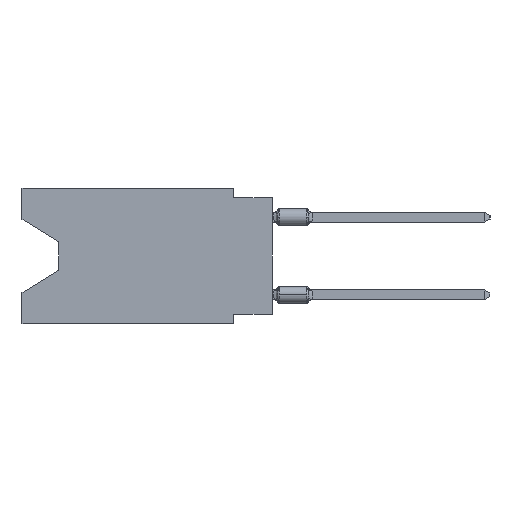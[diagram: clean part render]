
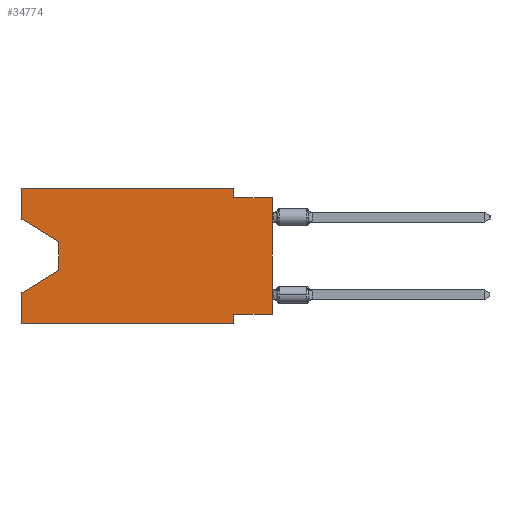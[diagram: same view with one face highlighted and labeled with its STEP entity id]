
A CAD part, left-side view. The second image highlights one B-rep face of the part: STEP entity #34774.
In plain terms, the highlighted planar face has unit normal (-1, 0, 0).
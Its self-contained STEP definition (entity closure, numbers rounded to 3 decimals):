
#83 = VERTEX_POINT ( 'NONE', #18799 ) ;
#604 = VECTOR ( 'NONE', #14084, 1000. ) ;
#1119 = CARTESIAN_POINT ( 'NONE',  ( 0., 0., -0.635 ) ) ;
#1254 = EDGE_CURVE ( 'NONE', #20307, #37080, #40412, .T. ) ;
#1419 = VECTOR ( 'NONE', #37211, 1000. ) ;
#2137 = VERTEX_POINT ( 'NONE', #32181 ) ;
#2532 = LINE ( 'NONE', #12318, #37651 ) ;
#3148 = CARTESIAN_POINT ( 'NONE',  ( 0., 16.383, -6.852 ) ) ;
#3188 = VERTEX_POINT ( 'NONE', #3148 ) ;
#3555 = VECTOR ( 'NONE', #18831, 1000. ) ;
#4075 = CARTESIAN_POINT ( 'NONE',  ( 0., 16.383, -8.89 ) ) ;
#4174 = VECTOR ( 'NONE', #4237, 1000. ) ;
#4237 = DIRECTION ( 'NONE',  ( 0., -0.855, -0.519 ) ) ;
#4525 = LINE ( 'NONE', #4075, #33786 ) ;
#4905 = VECTOR ( 'NONE', #16908, 1000. ) ;
#5247 = VERTEX_POINT ( 'NONE', #7346 ) ;
#5257 = ORIENTED_EDGE ( 'NONE', *, *, #14870, .T. ) ;
#6624 = CARTESIAN_POINT ( 'NONE',  ( 0., 2.54, -0.635 ) ) ;
#7346 = CARTESIAN_POINT ( 'NONE',  ( 0., 2.54, 0. ) ) ;
#7410 = ORIENTED_EDGE ( 'NONE', *, *, #8466, .T. ) ;
#8466 = EDGE_CURVE ( 'NONE', #13550, #20734, #4525, .T. ) ;
#8864 = PLANE ( 'NONE',  #40892 ) ;
#9084 = CARTESIAN_POINT ( 'NONE',  ( 0., 16.383, 0. ) ) ;
#10194 = CARTESIAN_POINT ( 'NONE',  ( 0., 16.383, 0. ) ) ;
#10317 = LINE ( 'NONE', #36293, #4905 ) ;
#10452 = EDGE_CURVE ( 'NONE', #15622, #37080, #33438, .T. ) ;
#10606 = CARTESIAN_POINT ( 'NONE',  ( 0., 13.97, -5.385 ) ) ;
#10803 = VERTEX_POINT ( 'NONE', #10194 ) ;
#10933 = LINE ( 'NONE', #39896, #32825 ) ;
#11164 = DIRECTION ( 'NONE',  ( 0., 0.855, -0.519 ) ) ;
#11846 = DIRECTION ( 'NONE',  ( 0., 0., -1. ) ) ;
#12318 = CARTESIAN_POINT ( 'NONE',  ( 0., 13.97, -3.505 ) ) ;
#12790 = VECTOR ( 'NONE', #40930, 1000. ) ;
#13257 = CARTESIAN_POINT ( 'NONE',  ( 0., 16.383, 0. ) ) ;
#13448 = LINE ( 'NONE', #13257, #41005 ) ;
#13550 = VERTEX_POINT ( 'NONE', #41225 ) ;
#14024 = LINE ( 'NONE', #20608, #4174 ) ;
#14041 = CARTESIAN_POINT ( 'NONE',  ( 0., 0., -0.635 ) ) ;
#14084 = DIRECTION ( 'NONE',  ( 0., -1., 0. ) ) ;
#14853 = CARTESIAN_POINT ( 'NONE',  ( 0., 0., 0. ) ) ;
#14870 = EDGE_CURVE ( 'NONE', #29955, #3188, #10933, .T. ) ;
#14952 = LINE ( 'NONE', #27925, #12790 ) ;
#15130 = EDGE_CURVE ( 'NONE', #13550, #3188, #13448, .T. ) ;
#15622 = VERTEX_POINT ( 'NONE', #6624 ) ;
#16066 = LINE ( 'NONE', #28405, #40468 ) ;
#16580 = ORIENTED_EDGE ( 'NONE', *, *, #21269, .F. ) ;
#16908 = DIRECTION ( 'NONE',  ( 0., 0., -1. ) ) ;
#18435 = VECTOR ( 'NONE', #35134, 1000. ) ;
#18553 = EDGE_LOOP ( 'NONE', ( #25967, #38367, #5257, #33891, #7410, #32512, #21854, #38124, #26604, #36884, #16580, #30901 ) ) ;
#18620 = LINE ( 'NONE', #31600, #3555 ) ;
#18799 = CARTESIAN_POINT ( 'NONE',  ( 0., 2.54, -8.255 ) ) ;
#18831 = DIRECTION ( 'NONE',  ( 0., 0., -1. ) ) ;
#20307 = VERTEX_POINT ( 'NONE', #37845 ) ;
#20608 = CARTESIAN_POINT ( 'NONE',  ( 0., 16.383, -2.038 ) ) ;
#20734 = VERTEX_POINT ( 'NONE', #40132 ) ;
#21269 = EDGE_CURVE ( 'NONE', #10803, #5247, #14952, .T. ) ;
#21854 = ORIENTED_EDGE ( 'NONE', *, *, #22989, .F. ) ;
#22989 = EDGE_CURVE ( 'NONE', #20307, #83, #16066, .T. ) ;
#24704 = CARTESIAN_POINT ( 'NONE',  ( 0., 16.383, -2.038 ) ) ;
#25323 = LINE ( 'NONE', #34289, #18435 ) ;
#25967 = ORIENTED_EDGE ( 'NONE', *, *, #33001, .T. ) ;
#26575 = EDGE_CURVE ( 'NONE', #5247, #15622, #18620, .T. ) ;
#26604 = ORIENTED_EDGE ( 'NONE', *, *, #10452, .F. ) ;
#27925 = CARTESIAN_POINT ( 'NONE',  ( 0., 16.383, 0. ) ) ;
#28405 = CARTESIAN_POINT ( 'NONE',  ( 0., 0., -8.255 ) ) ;
#29628 = DIRECTION ( 'NONE',  ( 0., 0., 1. ) ) ;
#29955 = VERTEX_POINT ( 'NONE', #10606 ) ;
#30462 = DIRECTION ( 'NONE',  ( 0., -1., 0. ) ) ;
#30901 = ORIENTED_EDGE ( 'NONE', *, *, #32720, .F. ) ;
#31600 = CARTESIAN_POINT ( 'NONE',  ( 0., 2.54, 0. ) ) ;
#32181 = CARTESIAN_POINT ( 'NONE',  ( 0., 13.97, -3.505 ) ) ;
#32512 = ORIENTED_EDGE ( 'NONE', *, *, #34872, .F. ) ;
#32720 = EDGE_CURVE ( 'NONE', #37687, #10803, #25323, .T. ) ;
#32825 = VECTOR ( 'NONE', #11164, 1000. ) ;
#33001 = EDGE_CURVE ( 'NONE', #37687, #2137, #14024, .T. ) ;
#33438 = LINE ( 'NONE', #1119, #604 ) ;
#33786 = VECTOR ( 'NONE', #30462, 1000. ) ;
#33891 = ORIENTED_EDGE ( 'NONE', *, *, #15130, .F. ) ;
#34289 = CARTESIAN_POINT ( 'NONE',  ( 0., 16.383, 0. ) ) ;
#34774 = ADVANCED_FACE ( 'NONE', ( #41638 ), #8864, .F. ) ;
#34872 = EDGE_CURVE ( 'NONE', #83, #20734, #10317, .T. ) ;
#35134 = DIRECTION ( 'NONE',  ( 0., 0., 1. ) ) ;
#36293 = CARTESIAN_POINT ( 'NONE',  ( 0., 2.54, -8.89 ) ) ;
#36884 = ORIENTED_EDGE ( 'NONE', *, *, #26575, .F. ) ;
#37080 = VERTEX_POINT ( 'NONE', #14041 ) ;
#37207 = EDGE_CURVE ( 'NONE', #2137, #29955, #2532, .T. ) ;
#37211 = DIRECTION ( 'NONE',  ( 0., 0., 1. ) ) ;
#37651 = VECTOR ( 'NONE', #37870, 1000. ) ;
#37687 = VERTEX_POINT ( 'NONE', #24704 ) ;
#37845 = CARTESIAN_POINT ( 'NONE',  ( 0., 0., -8.255 ) ) ;
#37870 = DIRECTION ( 'NONE',  ( 0., 0., -1. ) ) ;
#38124 = ORIENTED_EDGE ( 'NONE', *, *, #1254, .T. ) ;
#38367 = ORIENTED_EDGE ( 'NONE', *, *, #37207, .T. ) ;
#38423 = DIRECTION ( 'NONE',  ( 0., 1., 0. ) ) ;
#39896 = CARTESIAN_POINT ( 'NONE',  ( 0., 13.97, -5.385 ) ) ;
#40132 = CARTESIAN_POINT ( 'NONE',  ( 0., 2.54, -8.89 ) ) ;
#40412 = LINE ( 'NONE', #14853, #1419 ) ;
#40468 = VECTOR ( 'NONE', #38423, 1000. ) ;
#40892 = AXIS2_PLACEMENT_3D ( 'NONE', #9084, #40997, #11846 ) ;
#40930 = DIRECTION ( 'NONE',  ( 0., -1., 0. ) ) ;
#40997 = DIRECTION ( 'NONE',  ( 1., 0., 0. ) ) ;
#41005 = VECTOR ( 'NONE', #29628, 1000. ) ;
#41225 = CARTESIAN_POINT ( 'NONE',  ( 0., 16.383, -8.89 ) ) ;
#41638 = FACE_OUTER_BOUND ( 'NONE', #18553, .T. ) ;
